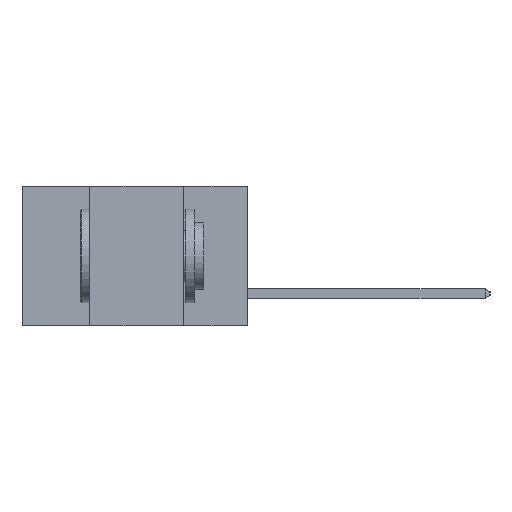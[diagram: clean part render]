
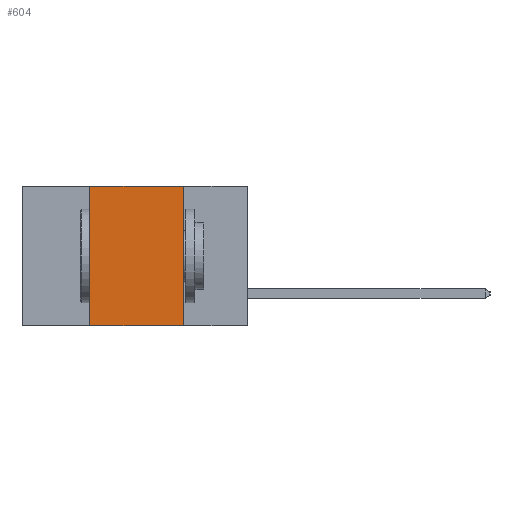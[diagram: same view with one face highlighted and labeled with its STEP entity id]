
A CAD part, left-side view. The second image highlights one B-rep face of the part: STEP entity #604.
In plain terms, the highlighted planar face has unit normal (-1, 0, 0).
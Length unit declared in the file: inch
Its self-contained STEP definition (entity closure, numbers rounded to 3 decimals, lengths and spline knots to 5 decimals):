
#245 = CARTESIAN_POINT ( 'NONE',  ( 0., 0.42, 0. ) ) ;
#604 = ADVANCED_FACE ( 'NONE', ( #9202 ), #5707, .F. ) ;
#752 = CARTESIAN_POINT ( 'NONE',  ( 0., 0.42, -0.37 ) ) ;
#922 = VECTOR ( 'NONE', #2062, 39.37008 ) ;
#997 = LINE ( 'NONE', #3498, #6752 ) ;
#1024 = CARTESIAN_POINT ( 'NONE',  ( 0., 0.6, 0. ) ) ;
#1036 = VERTEX_POINT ( 'NONE', #11437 ) ;
#1985 = ORIENTED_EDGE ( 'NONE', *, *, #12948, .F. ) ;
#2062 = DIRECTION ( 'NONE',  ( 0., -1., 0. ) ) ;
#2121 = ORIENTED_EDGE ( 'NONE', *, *, #12878, .F. ) ;
#2137 = ORIENTED_EDGE ( 'NONE', *, *, #6526, .F. ) ;
#2195 = ORIENTED_EDGE ( 'NONE', *, *, #5318, .T. ) ;
#2291 = CARTESIAN_POINT ( 'NONE',  ( 0., 0.6, 0. ) ) ;
#3498 = CARTESIAN_POINT ( 'NONE',  ( 0., 0.17, 0. ) ) ;
#4039 = LINE ( 'NONE', #11185, #922 ) ;
#5289 = AXIS2_PLACEMENT_3D ( 'NONE', #2291, #5870, #5867 ) ;
#5318 = EDGE_CURVE ( 'NONE', #5319, #12293, #4039, .T. ) ;
#5319 = VERTEX_POINT ( 'NONE', #752 ) ;
#5359 = CARTESIAN_POINT ( 'NONE',  ( 0., 0.17, 0. ) ) ;
#5707 = PLANE ( 'NONE',  #5289 ) ;
#5867 = DIRECTION ( 'NONE',  ( 0., 0., -1. ) ) ;
#5870 = DIRECTION ( 'NONE',  ( 1., 0., 0. ) ) ;
#6059 = EDGE_LOOP ( 'NONE', ( #1985, #2121, #2137, #2195 ) ) ;
#6526 = EDGE_CURVE ( 'NONE', #5319, #1036, #9057, .T. ) ;
#6752 = VECTOR ( 'NONE', #13203, 39.37008 ) ;
#8535 = DIRECTION ( 'NONE',  ( 0., 0., 1. ) ) ;
#9057 = LINE ( 'NONE', #245, #13917 ) ;
#9115 = CARTESIAN_POINT ( 'NONE',  ( 0., 0.17, -0.37 ) ) ;
#9202 = FACE_OUTER_BOUND ( 'NONE', #6059, .T. ) ;
#10312 = LINE ( 'NONE', #1024, #13068 ) ;
#10791 = VERTEX_POINT ( 'NONE', #5359 ) ;
#11185 = CARTESIAN_POINT ( 'NONE',  ( 0., 0.6, -0.37 ) ) ;
#11437 = CARTESIAN_POINT ( 'NONE',  ( 0., 0.42, 0. ) ) ;
#12293 = VERTEX_POINT ( 'NONE', #9115 ) ;
#12878 = EDGE_CURVE ( 'NONE', #1036, #10791, #10312, .T. ) ;
#12948 = EDGE_CURVE ( 'NONE', #10791, #12293, #997, .T. ) ;
#13068 = VECTOR ( 'NONE', #13114, 39.37008 ) ;
#13114 = DIRECTION ( 'NONE',  ( 0., -1., 0. ) ) ;
#13203 = DIRECTION ( 'NONE',  ( 0., 0., -1. ) ) ;
#13917 = VECTOR ( 'NONE', #8535, 39.37008 ) ;
